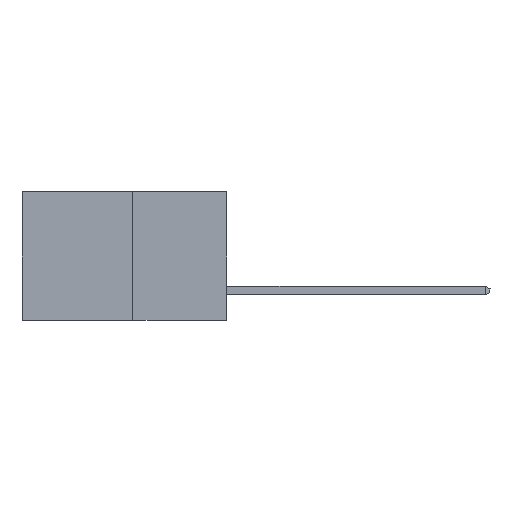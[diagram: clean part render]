
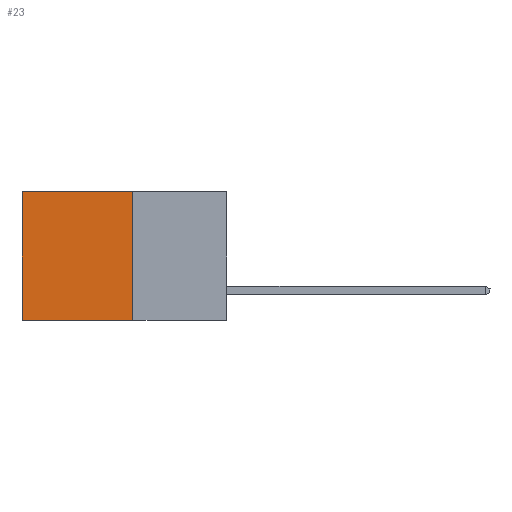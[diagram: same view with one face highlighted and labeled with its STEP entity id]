
A CAD part, left-side view. The second image highlights one B-rep face of the part: STEP entity #23.
In plain terms, the highlighted planar face has unit normal (-1, 0, 0).
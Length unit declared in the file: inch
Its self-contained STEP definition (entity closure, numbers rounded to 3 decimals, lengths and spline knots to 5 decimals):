
#20 = LINE ( 'NONE', #2452, #2527 ) ;
#23 = ADVANCED_FACE ( 'NONE', ( #6077 ), #4275, .F. ) ;
#275 = CARTESIAN_POINT ( 'NONE',  ( 0.277, 0.59, 0. ) ) ;
#440 = DIRECTION ( 'NONE',  ( 0., 0., -1. ) ) ;
#482 = CARTESIAN_POINT ( 'NONE',  ( 0.277, 0.27, -0.37 ) ) ;
#843 = VERTEX_POINT ( 'NONE', #275 ) ;
#1203 = CARTESIAN_POINT ( 'NONE',  ( 0.277, 0.27, -0.37 ) ) ;
#2452 = CARTESIAN_POINT ( 'NONE',  ( 0.277, 0.27, -0.37 ) ) ;
#2527 = VECTOR ( 'NONE', #5616, 39.37008 ) ;
#2995 = VECTOR ( 'NONE', #12144, 39.37008 ) ;
#3318 = LINE ( 'NONE', #482, #8527 ) ;
#4169 = DIRECTION ( 'NONE',  ( 1., 0., 0. ) ) ;
#4275 = PLANE ( 'NONE',  #9863 ) ;
#4397 = CARTESIAN_POINT ( 'NONE',  ( 0.277, 0.59, -0.37 ) ) ;
#4420 = VERTEX_POINT ( 'NONE', #12689 ) ;
#4441 = LINE ( 'NONE', #13130, #12884 ) ;
#5052 = ORIENTED_EDGE ( 'NONE', *, *, #5100, .F. ) ;
#5100 = EDGE_CURVE ( 'NONE', #4420, #12818, #3318, .T. ) ;
#5183 = EDGE_CURVE ( 'NONE', #4420, #843, #7881, .T. ) ;
#5616 = DIRECTION ( 'NONE',  ( 0., 1., 0. ) ) ;
#6077 = FACE_OUTER_BOUND ( 'NONE', #8067, .T. ) ;
#7805 = CARTESIAN_POINT ( 'NONE',  ( 0.277, 0.27, -0.37 ) ) ;
#7881 = LINE ( 'NONE', #12606, #2995 ) ;
#8067 = EDGE_LOOP ( 'NONE', ( #12508, #12831, #5052, #10488 ) ) ;
#8123 = DIRECTION ( 'NONE',  ( 0., 0., -1. ) ) ;
#8527 = VECTOR ( 'NONE', #440, 39.37008 ) ;
#9863 = AXIS2_PLACEMENT_3D ( 'NONE', #1203, #4169, #12808 ) ;
#10488 = ORIENTED_EDGE ( 'NONE', *, *, #5183, .T. ) ;
#11290 = EDGE_CURVE ( 'NONE', #12818, #11931, #20, .T. ) ;
#11931 = VERTEX_POINT ( 'NONE', #4397 ) ;
#12144 = DIRECTION ( 'NONE',  ( 0., 1., 0. ) ) ;
#12436 = EDGE_CURVE ( 'NONE', #843, #11931, #4441, .T. ) ;
#12508 = ORIENTED_EDGE ( 'NONE', *, *, #12436, .T. ) ;
#12606 = CARTESIAN_POINT ( 'NONE',  ( 0.277, 0.27, 0. ) ) ;
#12689 = CARTESIAN_POINT ( 'NONE',  ( 0.277, 0.27, 0. ) ) ;
#12808 = DIRECTION ( 'NONE',  ( 0., 0., -1. ) ) ;
#12818 = VERTEX_POINT ( 'NONE', #7805 ) ;
#12831 = ORIENTED_EDGE ( 'NONE', *, *, #11290, .F. ) ;
#12884 = VECTOR ( 'NONE', #8123, 39.37008 ) ;
#13130 = CARTESIAN_POINT ( 'NONE',  ( 0.277, 0.59, -0.37 ) ) ;
